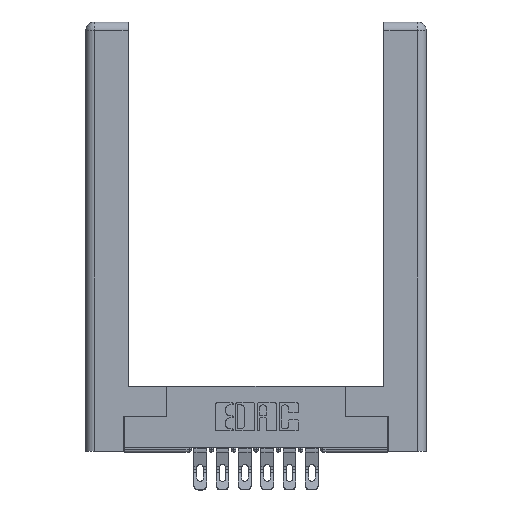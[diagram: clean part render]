
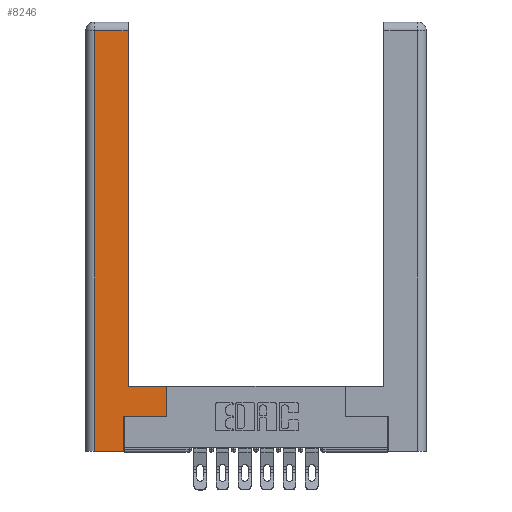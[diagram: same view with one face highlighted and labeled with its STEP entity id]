
A CAD part, top view. The second image highlights one B-rep face of the part: STEP entity #8246.
In plain terms, the highlighted planar face has unit normal (0, 0, 1).
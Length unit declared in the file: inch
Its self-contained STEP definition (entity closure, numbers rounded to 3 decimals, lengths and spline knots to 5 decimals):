
#75 = ORIENTED_EDGE ( 'NONE', *, *, #9554, .T. ) ;
#162 = LINE ( 'NONE', #9673, #2063 ) ;
#186 = CARTESIAN_POINT ( 'NONE',  ( 0.0615, 2.94, 0. ) ) ;
#230 = VECTOR ( 'NONE', #13620, 39.37008 ) ;
#337 = CARTESIAN_POINT ( 'NONE',  ( 0., 0., 0. ) ) ;
#671 = DIRECTION ( 'NONE',  ( 0., -1., 0. ) ) ;
#752 = EDGE_CURVE ( 'NONE', #2185, #9477, #5756, .T. ) ;
#849 = VECTOR ( 'NONE', #918, 39.37008 ) ;
#918 = DIRECTION ( 'NONE',  ( -1., 0., 0. ) ) ;
#971 = DIRECTION ( 'NONE',  ( 1., 0., 0. ) ) ;
#1512 = EDGE_CURVE ( 'NONE', #4336, #6480, #11891, .T. ) ;
#1947 = FACE_OUTER_BOUND ( 'NONE', #13344, .T. ) ;
#2063 = VECTOR ( 'NONE', #4423, 39.37008 ) ;
#2185 = VERTEX_POINT ( 'NONE', #4661 ) ;
#2310 = EDGE_CURVE ( 'NONE', #7170, #2185, #6766, .T. ) ;
#2341 = ORIENTED_EDGE ( 'NONE', *, *, #13602, .T. ) ;
#3183 = VECTOR ( 'NONE', #6664, 39.37008 ) ;
#3592 = ORIENTED_EDGE ( 'NONE', *, *, #13670, .T. ) ;
#4018 = CARTESIAN_POINT ( 'NONE',  ( 0.565, 0.245, 0. ) ) ;
#4091 = LINE ( 'NONE', #8109, #4593 ) ;
#4336 = VERTEX_POINT ( 'NONE', #11386 ) ;
#4392 = CARTESIAN_POINT ( 'NONE',  ( 0.0615, 0., 0. ) ) ;
#4423 = DIRECTION ( 'NONE',  ( 1., 0., 0. ) ) ;
#4593 = VECTOR ( 'NONE', #971, 39.37008 ) ;
#4609 = CARTESIAN_POINT ( 'NONE',  ( 0.565, 0.45, 0. ) ) ;
#4661 = CARTESIAN_POINT ( 'NONE',  ( 0.295, 2.94, 0. ) ) ;
#4758 = DIRECTION ( 'NONE',  ( -1., 0., 0. ) ) ;
#4760 = ORIENTED_EDGE ( 'NONE', *, *, #11505, .T. ) ;
#4978 = VERTEX_POINT ( 'NONE', #4392 ) ;
#5372 = CARTESIAN_POINT ( 'NONE',  ( 0.0615, 2.94, 0. ) ) ;
#5530 = ORIENTED_EDGE ( 'NONE', *, *, #1512, .T. ) ;
#5593 = ORIENTED_EDGE ( 'NONE', *, *, #9113, .T. ) ;
#5670 = LINE ( 'NONE', #8715, #8210 ) ;
#5756 = LINE ( 'NONE', #186, #3183 ) ;
#6076 = CARTESIAN_POINT ( 'NONE',  ( 0.295, 3., 0. ) ) ;
#6480 = VERTEX_POINT ( 'NONE', #11104 ) ;
#6664 = DIRECTION ( 'NONE',  ( -1., 0., 0. ) ) ;
#6766 = LINE ( 'NONE', #6076, #230 ) ;
#6886 = ORIENTED_EDGE ( 'NONE', *, *, #752, .T. ) ;
#7170 = VERTEX_POINT ( 'NONE', #8512 ) ;
#7539 = VERTEX_POINT ( 'NONE', #4018 ) ;
#7619 = CARTESIAN_POINT ( 'NONE',  ( 0.295, 0.45, 0. ) ) ;
#8109 = CARTESIAN_POINT ( 'NONE',  ( 0.265, 0., 0. ) ) ;
#8114 = VERTEX_POINT ( 'NONE', #4609 ) ;
#8210 = VECTOR ( 'NONE', #8616, 39.37008 ) ;
#8246 = ADVANCED_FACE ( 'NONE', ( #1947 ), #9296, .F. ) ;
#8505 = ORIENTED_EDGE ( 'NONE', *, *, #2310, .T. ) ;
#8512 = CARTESIAN_POINT ( 'NONE',  ( 0.295, 0.45, 0. ) ) ;
#8616 = DIRECTION ( 'NONE',  ( 0., 1., 0. ) ) ;
#8715 = CARTESIAN_POINT ( 'NONE',  ( 0.565, 0.45, 0. ) ) ;
#9113 = EDGE_CURVE ( 'NONE', #9477, #4978, #12667, .T. ) ;
#9258 = AXIS2_PLACEMENT_3D ( 'NONE', #337, #10187, #4758 ) ;
#9296 = PLANE ( 'NONE',  #9258 ) ;
#9463 = CARTESIAN_POINT ( 'NONE',  ( 0.265, 0.245, 0. ) ) ;
#9477 = VERTEX_POINT ( 'NONE', #5372 ) ;
#9552 = DIRECTION ( 'NONE',  ( 0., 1., 0. ) ) ;
#9554 = EDGE_CURVE ( 'NONE', #8114, #7170, #13159, .T. ) ;
#9673 = CARTESIAN_POINT ( 'NONE',  ( 0.565, 0.245, 0. ) ) ;
#9753 = VECTOR ( 'NONE', #671, 39.37008 ) ;
#10187 = DIRECTION ( 'NONE',  ( 0., 0., -1. ) ) ;
#10500 = CARTESIAN_POINT ( 'NONE',  ( 0.0615, 0., 0. ) ) ;
#10707 = VECTOR ( 'NONE', #9552, 39.37008 ) ;
#11104 = CARTESIAN_POINT ( 'NONE',  ( 0.265, 0.245, 0. ) ) ;
#11386 = CARTESIAN_POINT ( 'NONE',  ( 0.265, 0., 0. ) ) ;
#11505 = EDGE_CURVE ( 'NONE', #4978, #4336, #4091, .T. ) ;
#11891 = LINE ( 'NONE', #9463, #10707 ) ;
#12667 = LINE ( 'NONE', #10500, #9753 ) ;
#13159 = LINE ( 'NONE', #7619, #849 ) ;
#13344 = EDGE_LOOP ( 'NONE', ( #8505, #6886, #5593, #4760, #5530, #2341, #3592, #75 ) ) ;
#13602 = EDGE_CURVE ( 'NONE', #6480, #7539, #162, .T. ) ;
#13620 = DIRECTION ( 'NONE',  ( 0., 1., 0. ) ) ;
#13670 = EDGE_CURVE ( 'NONE', #7539, #8114, #5670, .T. ) ;
